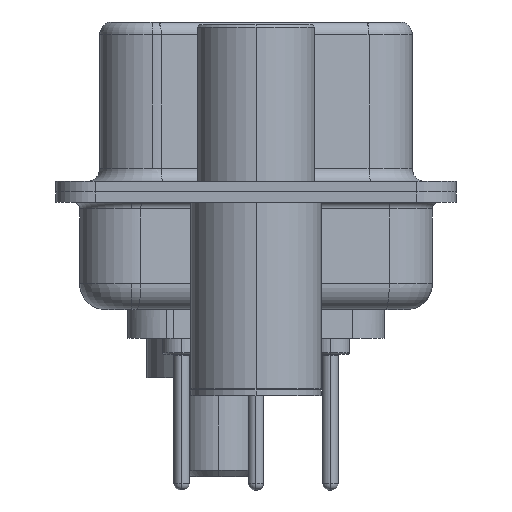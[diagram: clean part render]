
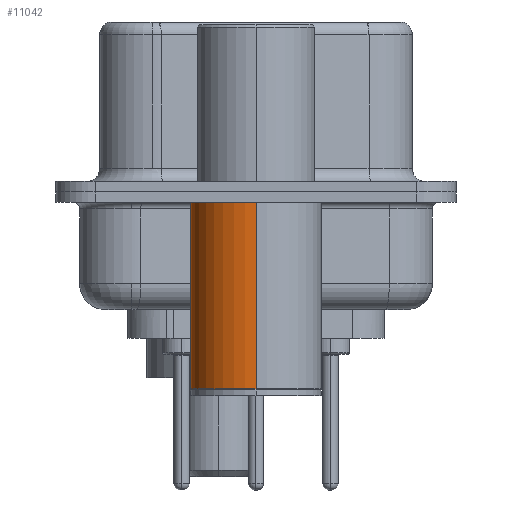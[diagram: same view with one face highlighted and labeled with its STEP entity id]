
A CAD part, left-side view. The second image highlights one B-rep face of the part: STEP entity #11042.
In plain terms, the highlighted cylindrical face has radius 2.5 mm (diameter 5 mm), a partial arc.
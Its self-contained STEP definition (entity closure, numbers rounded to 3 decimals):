
#795 = VERTEX_POINT ( 'NONE', #28420 ) ;
#948 = ORIENTED_EDGE ( 'NONE', *, *, #25321, .F. ) ;
#1099 = CARTESIAN_POINT ( 'NONE',  ( 0., 0., 0.581 ) ) ;
#1704 = CARTESIAN_POINT ( 'NONE',  ( -2.5, 0., 0.581 ) ) ;
#2700 = EDGE_CURVE ( 'NONE', #4246, #10642, #21125, .T. ) ;
#3909 = FACE_OUTER_BOUND ( 'NONE', #12041, .T. ) ;
#3977 = DIRECTION ( 'NONE',  ( 0., 0., 1. ) ) ;
#4246 = VERTEX_POINT ( 'NONE', #26274 ) ;
#5212 = VECTOR ( 'NONE', #32290, 1000. ) ;
#7334 = CARTESIAN_POINT ( 'NONE',  ( 0., 0., -7.525 ) ) ;
#8556 = CARTESIAN_POINT ( 'NONE',  ( -2.5, 0., -0.4 ) ) ;
#9837 = DIRECTION ( 'NONE',  ( 0., 0., 1. ) ) ;
#10183 = DIRECTION ( 'NONE',  ( 1., 0., 0. ) ) ;
#10642 = VERTEX_POINT ( 'NONE', #13414 ) ;
#10797 = ORIENTED_EDGE ( 'NONE', *, *, #2700, .F. ) ;
#11042 = ADVANCED_FACE ( 'NONE', ( #3909 ), #18979, .T. ) ;
#12041 = EDGE_LOOP ( 'NONE', ( #23522, #19058, #948, #10797 ) ) ;
#12275 = VERTEX_POINT ( 'NONE', #8556 ) ;
#12389 = DIRECTION ( 'NONE',  ( 1., 0., 0. ) ) ;
#13251 = EDGE_CURVE ( 'NONE', #4246, #795, #13579, .T. ) ;
#13414 = CARTESIAN_POINT ( 'NONE',  ( 2.5, 0., -0.4 ) ) ;
#13579 = CIRCLE ( 'NONE', #26223, 2.5 ) ;
#18979 = CYLINDRICAL_SURFACE ( 'NONE', #29904, 2.5 ) ;
#19058 = ORIENTED_EDGE ( 'NONE', *, *, #32777, .T. ) ;
#21125 = LINE ( 'NONE', #34513, #5212 ) ;
#21755 = AXIS2_PLACEMENT_3D ( 'NONE', #26766, #9837, #29582 ) ;
#23522 = ORIENTED_EDGE ( 'NONE', *, *, #13251, .T. ) ;
#25321 = EDGE_CURVE ( 'NONE', #10642, #12275, #31053, .T. ) ;
#26223 = AXIS2_PLACEMENT_3D ( 'NONE', #7334, #27112, #10183 ) ;
#26274 = CARTESIAN_POINT ( 'NONE',  ( 2.5, 0., -7.525 ) ) ;
#26298 = VECTOR ( 'NONE', #35480, 1000. ) ;
#26766 = CARTESIAN_POINT ( 'NONE',  ( 0., 0., -0.4 ) ) ;
#27112 = DIRECTION ( 'NONE',  ( 0., 0., 1. ) ) ;
#28420 = CARTESIAN_POINT ( 'NONE',  ( -2.5, 0., -7.525 ) ) ;
#29582 = DIRECTION ( 'NONE',  ( 1., 0., 0. ) ) ;
#29904 = AXIS2_PLACEMENT_3D ( 'NONE', #1099, #3977, #12389 ) ;
#31053 = CIRCLE ( 'NONE', #21755, 2.5 ) ;
#32290 = DIRECTION ( 'NONE',  ( 0., 0., 1. ) ) ;
#32777 = EDGE_CURVE ( 'NONE', #795, #12275, #34582, .T. ) ;
#34513 = CARTESIAN_POINT ( 'NONE',  ( 2.5, 0., 0.581 ) ) ;
#34582 = LINE ( 'NONE', #1704, #26298 ) ;
#35480 = DIRECTION ( 'NONE',  ( 0., 0., 1. ) ) ;
